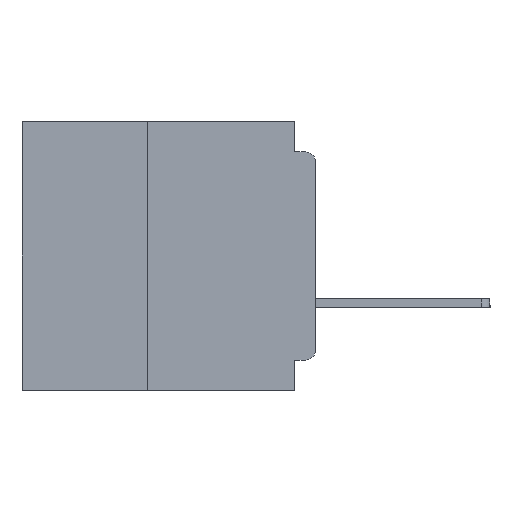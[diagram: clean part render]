
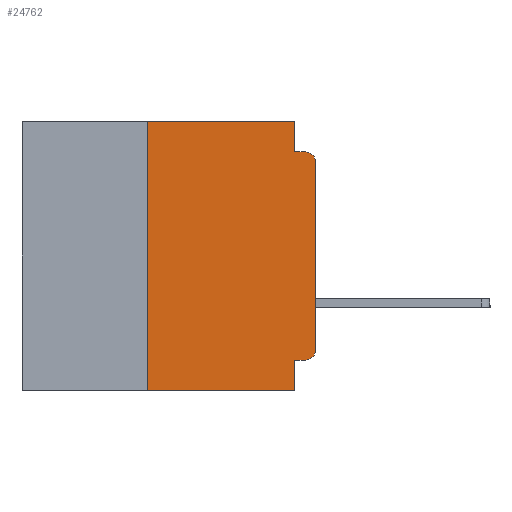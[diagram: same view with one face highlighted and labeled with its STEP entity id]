
A CAD part, left-side view. The second image highlights one B-rep face of the part: STEP entity #24762.
In plain terms, the highlighted planar face has unit normal (-1, 0, 0).
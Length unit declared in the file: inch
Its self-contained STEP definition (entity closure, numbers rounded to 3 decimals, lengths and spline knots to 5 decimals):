
#1228 = DIRECTION ( 'NONE',  ( 0., 0., -1. ) ) ;
#1487 = EDGE_CURVE ( 'NONE', #11538, #4438, #22758, .T. ) ;
#1710 = VECTOR ( 'NONE', #41553, 39.37008 ) ;
#1876 = ORIENTED_EDGE ( 'NONE', *, *, #15142, .T. ) ;
#2514 = VERTEX_POINT ( 'NONE', #6837 ) ;
#2647 = DIRECTION ( 'NONE',  ( 0., 0., 1. ) ) ;
#2866 = EDGE_CURVE ( 'NONE', #4438, #32782, #36854, .T. ) ;
#3825 = PLANE ( 'NONE',  #9781 ) ;
#4109 = ORIENTED_EDGE ( 'NONE', *, *, #8430, .T. ) ;
#4214 = VERTEX_POINT ( 'NONE', #15168 ) ;
#4438 = VERTEX_POINT ( 'NONE', #16455 ) ;
#5883 = EDGE_CURVE ( 'NONE', #2514, #40866, #39458, .T. ) ;
#5969 = DIRECTION ( 'NONE',  ( -1., 0., 0. ) ) ;
#6515 = VECTOR ( 'NONE', #18442, 39.37008 ) ;
#6715 = ORIENTED_EDGE ( 'NONE', *, *, #1487, .F. ) ;
#6837 = CARTESIAN_POINT ( 'NONE',  ( 0., 0.25, -0.4 ) ) ;
#6841 = VERTEX_POINT ( 'NONE', #28641 ) ;
#7636 = CARTESIAN_POINT ( 'NONE',  ( 0., 0., -0.045 ) ) ;
#7894 = CARTESIAN_POINT ( 'NONE',  ( 0., 0.25, -0.4 ) ) ;
#8430 = EDGE_CURVE ( 'NONE', #11538, #4214, #31233, .T. ) ;
#8798 = VECTOR ( 'NONE', #15256, 39.37008 ) ;
#9746 = VECTOR ( 'NONE', #10962, 39.37008 ) ;
#9781 = AXIS2_PLACEMENT_3D ( 'NONE', #30305, #10631, #33502 ) ;
#10403 = ORIENTED_EDGE ( 'NONE', *, *, #39113, .F. ) ;
#10631 = DIRECTION ( 'NONE',  ( 1., 0., 0. ) ) ;
#10962 = DIRECTION ( 'NONE',  ( 0., 0., -1. ) ) ;
#11063 = CARTESIAN_POINT ( 'NONE',  ( 0., 0.031, -0.4 ) ) ;
#11075 = FACE_OUTER_BOUND ( 'NONE', #17409, .T. ) ;
#11167 = EDGE_CURVE ( 'NONE', #33927, #24649, #14686, .T. ) ;
#11420 = ORIENTED_EDGE ( 'NONE', *, *, #33384, .F. ) ;
#11538 = VERTEX_POINT ( 'NONE', #29541 ) ;
#11812 = CIRCLE ( 'NONE', #21671, 0.015 ) ;
#12606 = VECTOR ( 'NONE', #27445, 39.37008 ) ;
#13077 = CARTESIAN_POINT ( 'NONE',  ( 0., 0.015, -0.045 ) ) ;
#13083 = CARTESIAN_POINT ( 'NONE',  ( 0., 0.437, 0. ) ) ;
#14686 = LINE ( 'NONE', #7636, #12606 ) ;
#15040 = CARTESIAN_POINT ( 'NONE',  ( 0., 0., -0.355 ) ) ;
#15142 = EDGE_CURVE ( 'NONE', #6841, #24649, #11812, .T. ) ;
#15168 = CARTESIAN_POINT ( 'NONE',  ( 0., 0., -0.34 ) ) ;
#15256 = DIRECTION ( 'NONE',  ( 0., 1., 0. ) ) ;
#15405 = LINE ( 'NONE', #28184, #6515 ) ;
#16455 = CARTESIAN_POINT ( 'NONE',  ( 0., 0.031, -0.355 ) ) ;
#17409 = EDGE_LOOP ( 'NONE', ( #32861, #1876, #25780, #11420, #10403, #24305, #34990, #37979, #6715, #4109 ) ) ;
#18442 = DIRECTION ( 'NONE',  ( 0., -1., 0. ) ) ;
#19314 = CARTESIAN_POINT ( 'NONE',  ( 0., 0., 0. ) ) ;
#20326 = VECTOR ( 'NONE', #35942, 39.37008 ) ;
#21241 = DIRECTION ( 'NONE',  ( -1., 0., 0. ) ) ;
#21671 = AXIS2_PLACEMENT_3D ( 'NONE', #25807, #5969, #29117 ) ;
#22428 = VERTEX_POINT ( 'NONE', #28543 ) ;
#22758 = LINE ( 'NONE', #15040, #8798 ) ;
#22889 = AXIS2_PLACEMENT_3D ( 'NONE', #40569, #21241, #1228 ) ;
#24305 = ORIENTED_EDGE ( 'NONE', *, *, #5883, .F. ) ;
#24649 = VERTEX_POINT ( 'NONE', #13077 ) ;
#24762 = ADVANCED_FACE ( 'NONE', ( #11075 ), #3825, .F. ) ;
#24904 = CARTESIAN_POINT ( 'NONE',  ( 0., 0.031, -0.045 ) ) ;
#25563 = CARTESIAN_POINT ( 'NONE',  ( 0., 0.031, -0.4 ) ) ;
#25780 = ORIENTED_EDGE ( 'NONE', *, *, #11167, .F. ) ;
#25807 = CARTESIAN_POINT ( 'NONE',  ( 0., 0.015, -0.06 ) ) ;
#26404 = EDGE_CURVE ( 'NONE', #4214, #6841, #32394, .T. ) ;
#27445 = DIRECTION ( 'NONE',  ( 0., -1., 0. ) ) ;
#28184 = CARTESIAN_POINT ( 'NONE',  ( 0., 0.437, -0.4 ) ) ;
#28214 = LINE ( 'NONE', #38343, #1710 ) ;
#28543 = CARTESIAN_POINT ( 'NONE',  ( 0., 0.031, 0. ) ) ;
#28641 = CARTESIAN_POINT ( 'NONE',  ( 0., 0., -0.06 ) ) ;
#28742 = CARTESIAN_POINT ( 'NONE',  ( 0., 0.25, 0. ) ) ;
#28996 = LINE ( 'NONE', #13083, #20326 ) ;
#29117 = DIRECTION ( 'NONE',  ( 0., 0., -1. ) ) ;
#29541 = CARTESIAN_POINT ( 'NONE',  ( 0., 0.015, -0.355 ) ) ;
#30305 = CARTESIAN_POINT ( 'NONE',  ( 0., 0.437, 0. ) ) ;
#30947 = VECTOR ( 'NONE', #37399, 39.37008 ) ;
#31233 = CIRCLE ( 'NONE', #22889, 0.015 ) ;
#31425 = VECTOR ( 'NONE', #2647, 39.37008 ) ;
#32394 = LINE ( 'NONE', #19314, #31425 ) ;
#32640 = EDGE_CURVE ( 'NONE', #2514, #32782, #15405, .T. ) ;
#32782 = VERTEX_POINT ( 'NONE', #25563 ) ;
#32861 = ORIENTED_EDGE ( 'NONE', *, *, #26404, .T. ) ;
#33384 = EDGE_CURVE ( 'NONE', #22428, #33927, #28214, .T. ) ;
#33502 = DIRECTION ( 'NONE',  ( 0., 0., -1. ) ) ;
#33927 = VERTEX_POINT ( 'NONE', #24904 ) ;
#34990 = ORIENTED_EDGE ( 'NONE', *, *, #32640, .T. ) ;
#35942 = DIRECTION ( 'NONE',  ( 0., -1., 0. ) ) ;
#36854 = LINE ( 'NONE', #11063, #9746 ) ;
#37399 = DIRECTION ( 'NONE',  ( 0., 0., 1. ) ) ;
#37979 = ORIENTED_EDGE ( 'NONE', *, *, #2866, .F. ) ;
#38343 = CARTESIAN_POINT ( 'NONE',  ( 0., 0.031, 0. ) ) ;
#39113 = EDGE_CURVE ( 'NONE', #40866, #22428, #28996, .T. ) ;
#39458 = LINE ( 'NONE', #7894, #30947 ) ;
#40569 = CARTESIAN_POINT ( 'NONE',  ( 0., 0.015, -0.34 ) ) ;
#40866 = VERTEX_POINT ( 'NONE', #28742 ) ;
#41553 = DIRECTION ( 'NONE',  ( 0., 0., -1. ) ) ;
